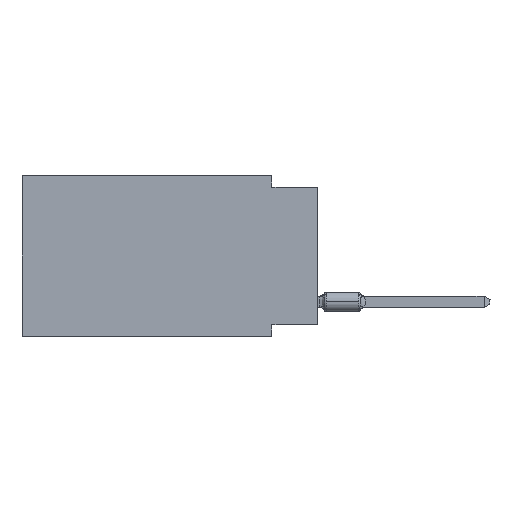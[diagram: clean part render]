
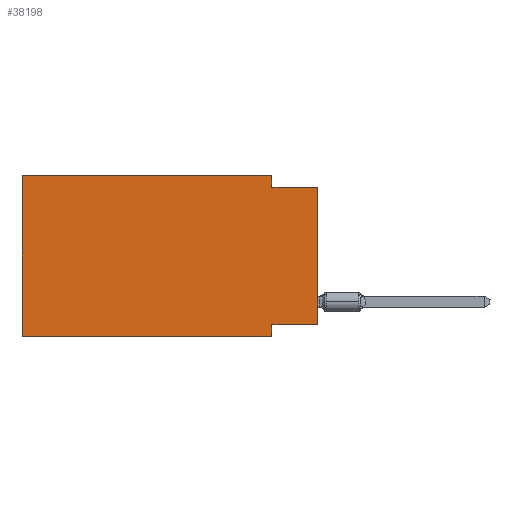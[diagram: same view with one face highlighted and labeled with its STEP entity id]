
A CAD part, left-side view. The second image highlights one B-rep face of the part: STEP entity #38198.
In plain terms, the highlighted planar face has unit normal (-1, 0, 0).
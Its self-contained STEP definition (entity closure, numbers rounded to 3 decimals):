
#3204 = EDGE_CURVE ( 'NONE', #38462, #46212, #36828, .T. ) ;
#4396 = DIRECTION ( 'NONE',  ( 0., 0., -1. ) ) ;
#4790 = CARTESIAN_POINT ( 'NONE',  ( 0., 2.54, -8.89 ) ) ;
#5091 = EDGE_CURVE ( 'NONE', #46212, #70477, #40746, .T. ) ;
#5737 = EDGE_CURVE ( 'NONE', #32861, #43316, #76114, .T. ) ;
#5980 = FACE_OUTER_BOUND ( 'NONE', #65824, .T. ) ;
#6673 = ORIENTED_EDGE ( 'NONE', *, *, #24986, .T. ) ;
#10486 = CARTESIAN_POINT ( 'NONE',  ( 0., 0., -0.635 ) ) ;
#13626 = DIRECTION ( 'NONE',  ( 0., 0., -1. ) ) ;
#14639 = DIRECTION ( 'NONE',  ( 0., 1., 0. ) ) ;
#15127 = CARTESIAN_POINT ( 'NONE',  ( 0., 2.54, 0. ) ) ;
#15396 = AXIS2_PLACEMENT_3D ( 'NONE', #31444, #62562, #13626 ) ;
#16572 = VECTOR ( 'NONE', #61651, 1000. ) ;
#19072 = CARTESIAN_POINT ( 'NONE',  ( 0., 2.54, -8.89 ) ) ;
#20277 = VECTOR ( 'NONE', #46009, 1000. ) ;
#20954 = ORIENTED_EDGE ( 'NONE', *, *, #49481, .F. ) ;
#22515 = CARTESIAN_POINT ( 'NONE',  ( 0., 16.383, 0. ) ) ;
#23043 = DIRECTION ( 'NONE',  ( 0., -1., 0. ) ) ;
#23397 = LINE ( 'NONE', #4790, #43763 ) ;
#24798 = VERTEX_POINT ( 'NONE', #19072 ) ;
#24986 = EDGE_CURVE ( 'NONE', #32861, #79432, #51232, .T. ) ;
#27375 = VECTOR ( 'NONE', #45935, 1000. ) ;
#28209 = ORIENTED_EDGE ( 'NONE', *, *, #5091, .F. ) ;
#28212 = ORIENTED_EDGE ( 'NONE', *, *, #40920, .T. ) ;
#28501 = EDGE_CURVE ( 'NONE', #70477, #79432, #59419, .T. ) ;
#31444 = CARTESIAN_POINT ( 'NONE',  ( 0., 16.383, 0. ) ) ;
#32861 = VERTEX_POINT ( 'NONE', #63851 ) ;
#33436 = CARTESIAN_POINT ( 'NONE',  ( 0., 0., 0. ) ) ;
#34175 = ORIENTED_EDGE ( 'NONE', *, *, #3204, .F. ) ;
#35302 = ORIENTED_EDGE ( 'NONE', *, *, #67328, .F. ) ;
#36828 = LINE ( 'NONE', #73644, #48412 ) ;
#36973 = LINE ( 'NONE', #38156, #16572 ) ;
#38156 = CARTESIAN_POINT ( 'NONE',  ( 0., 16.383, 0. ) ) ;
#38198 = ADVANCED_FACE ( 'NONE', ( #5980 ), #43973, .F. ) ;
#38462 = VERTEX_POINT ( 'NONE', #22515 ) ;
#38903 = ORIENTED_EDGE ( 'NONE', *, *, #5737, .F. ) ;
#39869 = CARTESIAN_POINT ( 'NONE',  ( 0., 16.383, -8.89 ) ) ;
#40746 = LINE ( 'NONE', #64216, #20277 ) ;
#40920 = EDGE_CURVE ( 'NONE', #72989, #24798, #46745, .T. ) ;
#43316 = VERTEX_POINT ( 'NONE', #71536 ) ;
#43763 = VECTOR ( 'NONE', #4396, 1000. ) ;
#43973 = PLANE ( 'NONE',  #15396 ) ;
#44479 = CARTESIAN_POINT ( 'NONE',  ( 0., 0., -0.635 ) ) ;
#45935 = DIRECTION ( 'NONE',  ( 0., -1., 0. ) ) ;
#46009 = DIRECTION ( 'NONE',  ( 0., 0., -1. ) ) ;
#46212 = VERTEX_POINT ( 'NONE', #15127 ) ;
#46745 = LINE ( 'NONE', #39869, #27375 ) ;
#48412 = VECTOR ( 'NONE', #61909, 1000. ) ;
#48832 = CARTESIAN_POINT ( 'NONE',  ( 0., 2.54, -0.635 ) ) ;
#49481 = EDGE_CURVE ( 'NONE', #43316, #24798, #23397, .T. ) ;
#51232 = LINE ( 'NONE', #33436, #67883 ) ;
#55367 = CARTESIAN_POINT ( 'NONE',  ( 0., 16.383, -8.89 ) ) ;
#59419 = LINE ( 'NONE', #10486, #60379 ) ;
#60379 = VECTOR ( 'NONE', #23043, 1000. ) ;
#61651 = DIRECTION ( 'NONE',  ( 0., 0., 1. ) ) ;
#61909 = DIRECTION ( 'NONE',  ( 0., -1., 0. ) ) ;
#62562 = DIRECTION ( 'NONE',  ( 1., 0., 0. ) ) ;
#63851 = CARTESIAN_POINT ( 'NONE',  ( 0., 0., -8.255 ) ) ;
#64216 = CARTESIAN_POINT ( 'NONE',  ( 0., 2.54, 0. ) ) ;
#65824 = EDGE_LOOP ( 'NONE', ( #6673, #73893, #28209, #34175, #35302, #28212, #20954, #38903 ) ) ;
#67328 = EDGE_CURVE ( 'NONE', #72989, #38462, #36973, .T. ) ;
#67883 = VECTOR ( 'NONE', #75907, 1000. ) ;
#70043 = CARTESIAN_POINT ( 'NONE',  ( 0., 0., -8.255 ) ) ;
#70477 = VERTEX_POINT ( 'NONE', #48832 ) ;
#71536 = CARTESIAN_POINT ( 'NONE',  ( 0., 2.54, -8.255 ) ) ;
#72989 = VERTEX_POINT ( 'NONE', #55367 ) ;
#73644 = CARTESIAN_POINT ( 'NONE',  ( 0., 16.383, 0. ) ) ;
#73893 = ORIENTED_EDGE ( 'NONE', *, *, #28501, .F. ) ;
#75907 = DIRECTION ( 'NONE',  ( 0., 0., 1. ) ) ;
#76114 = LINE ( 'NONE', #70043, #77101 ) ;
#77101 = VECTOR ( 'NONE', #14639, 1000. ) ;
#79432 = VERTEX_POINT ( 'NONE', #44479 ) ;
